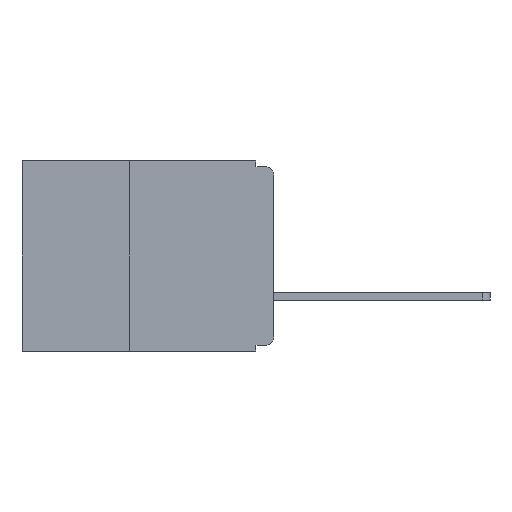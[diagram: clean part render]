
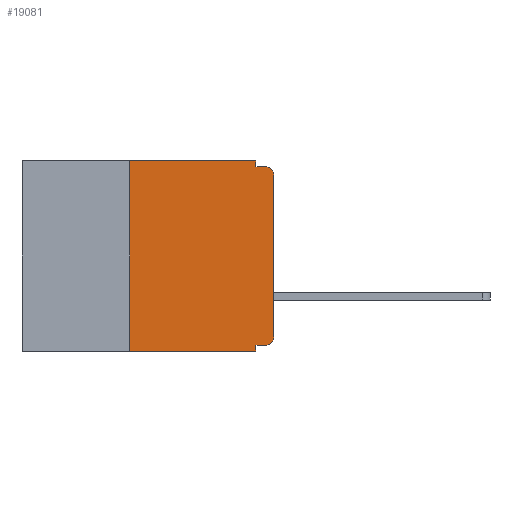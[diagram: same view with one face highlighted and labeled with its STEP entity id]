
A CAD part, left-side view. The second image highlights one B-rep face of the part: STEP entity #19081.
In plain terms, the highlighted planar face has unit normal (-1, 0, 0).
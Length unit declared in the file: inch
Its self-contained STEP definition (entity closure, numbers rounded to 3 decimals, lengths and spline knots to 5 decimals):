
#288 = DIRECTION ( 'NONE',  ( -1., 0., 0. ) ) ;
#647 = DIRECTION ( 'NONE',  ( 0., -1., 0. ) ) ;
#848 = VERTEX_POINT ( 'NONE', #22671 ) ;
#1086 = EDGE_CURVE ( 'NONE', #6076, #6409, #4352, .T. ) ;
#1263 = ORIENTED_EDGE ( 'NONE', *, *, #14677, .T. ) ;
#1975 = VECTOR ( 'NONE', #17117, 39.37008 ) ;
#1990 = VECTOR ( 'NONE', #647, 39.37008 ) ;
#2516 = ORIENTED_EDGE ( 'NONE', *, *, #14258, .F. ) ;
#2838 = VERTEX_POINT ( 'NONE', #7790 ) ;
#3118 = ORIENTED_EDGE ( 'NONE', *, *, #8555, .F. ) ;
#3275 = ORIENTED_EDGE ( 'NONE', *, *, #10040, .F. ) ;
#3773 = VECTOR ( 'NONE', #7662, 39.37008 ) ;
#4352 = CIRCLE ( 'NONE', #8219, 0.015 ) ;
#4544 = LINE ( 'NONE', #16800, #21448 ) ;
#4710 = EDGE_CURVE ( 'NONE', #14947, #2838, #5443, .T. ) ;
#4776 = CARTESIAN_POINT ( 'NONE',  ( 0., 0.031, 0. ) ) ;
#5105 = CARTESIAN_POINT ( 'NONE',  ( 0., 0.015, -0.305 ) ) ;
#5443 = LINE ( 'NONE', #11022, #28162 ) ;
#6076 = VERTEX_POINT ( 'NONE', #21072 ) ;
#6126 = ORIENTED_EDGE ( 'NONE', *, *, #4710, .F. ) ;
#6160 = CARTESIAN_POINT ( 'NONE',  ( 0., 0.031, -0.33 ) ) ;
#6324 = CARTESIAN_POINT ( 'NONE',  ( 0., 0., -0.305 ) ) ;
#6409 = VERTEX_POINT ( 'NONE', #16622 ) ;
#7143 = DIRECTION ( 'NONE',  ( 1., 0., 0. ) ) ;
#7323 = ORIENTED_EDGE ( 'NONE', *, *, #18528, .T. ) ;
#7351 = DIRECTION ( 'NONE',  ( 0., 0., -1. ) ) ;
#7662 = DIRECTION ( 'NONE',  ( 0., -1., 0. ) ) ;
#7790 = CARTESIAN_POINT ( 'NONE',  ( 0., 0.25, 0. ) ) ;
#7893 = VERTEX_POINT ( 'NONE', #27812 ) ;
#8091 = VERTEX_POINT ( 'NONE', #15179 ) ;
#8219 = AXIS2_PLACEMENT_3D ( 'NONE', #28549, #288, #21606 ) ;
#8555 = EDGE_CURVE ( 'NONE', #9154, #27358, #4544, .T. ) ;
#9154 = VERTEX_POINT ( 'NONE', #25441 ) ;
#10040 = EDGE_CURVE ( 'NONE', #7893, #8091, #27552, .T. ) ;
#10356 = LINE ( 'NONE', #25283, #3773 ) ;
#10423 = CARTESIAN_POINT ( 'NONE',  ( 0., 0.25, -0.33 ) ) ;
#10500 = DIRECTION ( 'NONE',  ( 0., 0., 1. ) ) ;
#10882 = EDGE_CURVE ( 'NONE', #27358, #848, #16846, .T. ) ;
#11022 = CARTESIAN_POINT ( 'NONE',  ( 0., 0.25, -0.33 ) ) ;
#11684 = CARTESIAN_POINT ( 'NONE',  ( 0., 0.437, -0.33 ) ) ;
#11703 = VECTOR ( 'NONE', #12834, 39.37008 ) ;
#12834 = DIRECTION ( 'NONE',  ( 0., 0., -1. ) ) ;
#13153 = ORIENTED_EDGE ( 'NONE', *, *, #22130, .T. ) ;
#13696 = PLANE ( 'NONE',  #14780 ) ;
#14258 = EDGE_CURVE ( 'NONE', #8091, #6409, #10356, .T. ) ;
#14677 = EDGE_CURVE ( 'NONE', #9154, #17421, #21357, .T. ) ;
#14780 = AXIS2_PLACEMENT_3D ( 'NONE', #26877, #7143, #22595 ) ;
#14947 = VERTEX_POINT ( 'NONE', #10423 ) ;
#14974 = CARTESIAN_POINT ( 'NONE',  ( 0., 0.437, 0. ) ) ;
#15179 = CARTESIAN_POINT ( 'NONE',  ( 0., 0.031, -0.01 ) ) ;
#15585 = EDGE_CURVE ( 'NONE', #2838, #7893, #19604, .T. ) ;
#15816 = VECTOR ( 'NONE', #26737, 39.37008 ) ;
#16084 = CARTESIAN_POINT ( 'NONE',  ( 0., 0.031, -0.32 ) ) ;
#16324 = VECTOR ( 'NONE', #19560, 39.37008 ) ;
#16622 = CARTESIAN_POINT ( 'NONE',  ( 0., 0.015, -0.01 ) ) ;
#16800 = CARTESIAN_POINT ( 'NONE',  ( 0., 0., -0.32 ) ) ;
#16846 = LINE ( 'NONE', #6160, #11703 ) ;
#17016 = LINE ( 'NONE', #26102, #16324 ) ;
#17117 = DIRECTION ( 'NONE',  ( 0., -1., 0. ) ) ;
#17421 = VERTEX_POINT ( 'NONE', #6324 ) ;
#18259 = LINE ( 'NONE', #11684, #1990 ) ;
#18528 = EDGE_CURVE ( 'NONE', #17421, #6076, #17016, .T. ) ;
#19028 = DIRECTION ( 'NONE',  ( 0., 1., 0. ) ) ;
#19081 = ADVANCED_FACE ( 'NONE', ( #19400 ), #13696, .F. ) ;
#19400 = FACE_OUTER_BOUND ( 'NONE', #25399, .T. ) ;
#19560 = DIRECTION ( 'NONE',  ( 0., 0., 1. ) ) ;
#19604 = LINE ( 'NONE', #14974, #1975 ) ;
#20429 = ORIENTED_EDGE ( 'NONE', *, *, #15585, .F. ) ;
#20528 = DIRECTION ( 'NONE',  ( -1., 0., 0. ) ) ;
#21072 = CARTESIAN_POINT ( 'NONE',  ( 0., 0., -0.025 ) ) ;
#21357 = CIRCLE ( 'NONE', #21711, 0.015 ) ;
#21448 = VECTOR ( 'NONE', #19028, 39.37008 ) ;
#21606 = DIRECTION ( 'NONE',  ( 0., 0., -1. ) ) ;
#21711 = AXIS2_PLACEMENT_3D ( 'NONE', #5105, #20528, #7351 ) ;
#22130 = EDGE_CURVE ( 'NONE', #14947, #848, #18259, .T. ) ;
#22595 = DIRECTION ( 'NONE',  ( 0., 0., -1. ) ) ;
#22671 = CARTESIAN_POINT ( 'NONE',  ( 0., 0.031, -0.33 ) ) ;
#24120 = ORIENTED_EDGE ( 'NONE', *, *, #1086, .T. ) ;
#25283 = CARTESIAN_POINT ( 'NONE',  ( 0., 0., -0.01 ) ) ;
#25399 = EDGE_LOOP ( 'NONE', ( #7323, #24120, #2516, #3275, #20429, #6126, #13153, #26969, #3118, #1263 ) ) ;
#25441 = CARTESIAN_POINT ( 'NONE',  ( 0., 0.015, -0.32 ) ) ;
#26102 = CARTESIAN_POINT ( 'NONE',  ( 0., 0., 0. ) ) ;
#26737 = DIRECTION ( 'NONE',  ( 0., 0., -1. ) ) ;
#26877 = CARTESIAN_POINT ( 'NONE',  ( 0., 0.437, 0. ) ) ;
#26969 = ORIENTED_EDGE ( 'NONE', *, *, #10882, .F. ) ;
#27358 = VERTEX_POINT ( 'NONE', #16084 ) ;
#27552 = LINE ( 'NONE', #4776, #15816 ) ;
#27812 = CARTESIAN_POINT ( 'NONE',  ( 0., 0.031, 0. ) ) ;
#28162 = VECTOR ( 'NONE', #10500, 39.37008 ) ;
#28549 = CARTESIAN_POINT ( 'NONE',  ( 0., 0.015, -0.025 ) ) ;
